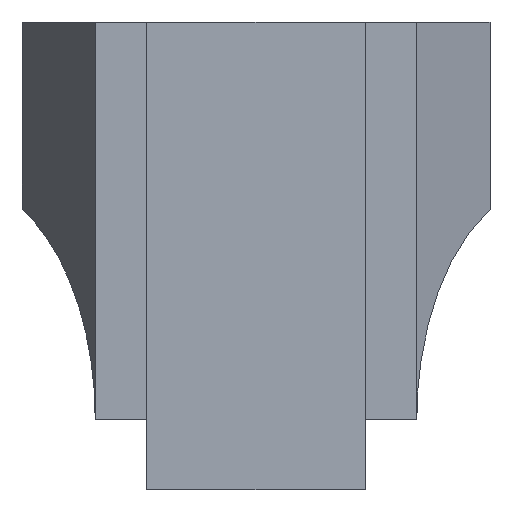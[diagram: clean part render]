
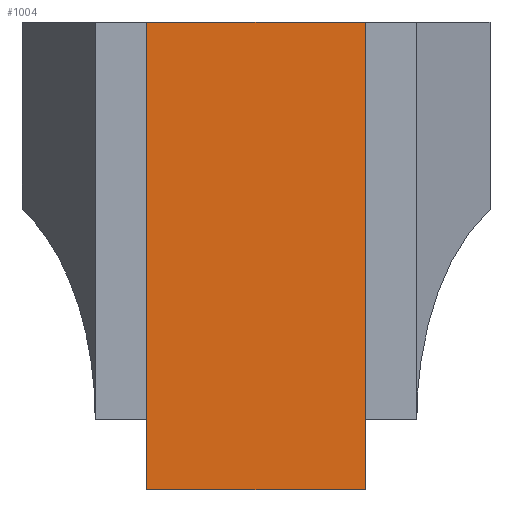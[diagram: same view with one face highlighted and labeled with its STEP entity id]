
A CAD part, front view. The second image highlights one B-rep face of the part: STEP entity #1004.
In plain terms, the highlighted planar face has unit normal (0, -1, 0).
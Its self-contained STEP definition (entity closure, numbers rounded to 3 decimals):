
#1004 = ADVANCED_FACE ( 'NONE', ( #13963 ), #10595, .T. ) ;
#1684 = CARTESIAN_POINT ( 'NONE',  ( 8.763, -36.779, -37.465 ) ) ;
#1995 = DIRECTION ( 'NONE',  ( 1., 0., 0. ) ) ;
#3786 = ORIENTED_EDGE ( 'NONE', *, *, #6204, .T. ) ;
#3848 = ORIENTED_EDGE ( 'NONE', *, *, #23478, .T. ) ;
#3893 = ORIENTED_EDGE ( 'NONE', *, *, #6611, .F. ) ;
#3922 = ORIENTED_EDGE ( 'NONE', *, *, #6567, .F. ) ;
#5533 = VECTOR ( 'NONE', #12416, 1000. ) ;
#5740 = EDGE_LOOP ( 'NONE', ( #3922, #3893, #3848, #3786 ) ) ;
#5918 = VERTEX_POINT ( 'NONE', #21819 ) ;
#6204 = EDGE_CURVE ( 'NONE', #5918, #16472, #19952, .T. ) ;
#6257 = VECTOR ( 'NONE', #18280, 1000. ) ;
#6567 = EDGE_CURVE ( 'NONE', #6609, #16472, #23216, .T. ) ;
#6609 = VERTEX_POINT ( 'NONE', #12443 ) ;
#6611 = EDGE_CURVE ( 'NONE', #12448, #6609, #9353, .T. ) ;
#9353 = LINE ( 'NONE', #12409, #25086 ) ;
#10561 = DIRECTION ( 'NONE',  ( 0., 0., -1. ) ) ;
#10587 = DIRECTION ( 'NONE',  ( 0., -1., 0. ) ) ;
#10595 = PLANE ( 'NONE',  #22796 ) ;
#10672 = CARTESIAN_POINT ( 'NONE',  ( 8.763, -36.779, -37.465 ) ) ;
#12132 = CARTESIAN_POINT ( 'NONE',  ( 8.763, -36.779, 0. ) ) ;
#12409 = CARTESIAN_POINT ( 'NONE',  ( -8.763, -36.779, -37.465 ) ) ;
#12416 = DIRECTION ( 'NONE',  ( 1., 0., 0. ) ) ;
#12443 = CARTESIAN_POINT ( 'NONE',  ( -8.763, -36.779, 0. ) ) ;
#12448 = VERTEX_POINT ( 'NONE', #17926 ) ;
#12679 = CARTESIAN_POINT ( 'NONE',  ( 8.763, -36.779, 0. ) ) ;
#13963 = FACE_OUTER_BOUND ( 'NONE', #5740, .T. ) ;
#14083 = LINE ( 'NONE', #26659, #16560 ) ;
#16472 = VERTEX_POINT ( 'NONE', #12132 ) ;
#16560 = VECTOR ( 'NONE', #1995, 1000. ) ;
#17926 = CARTESIAN_POINT ( 'NONE',  ( -8.763, -36.779, -37.465 ) ) ;
#18280 = DIRECTION ( 'NONE',  ( 0., 0., 1. ) ) ;
#19952 = LINE ( 'NONE', #1684, #6257 ) ;
#21819 = CARTESIAN_POINT ( 'NONE',  ( 8.763, -36.779, -37.465 ) ) ;
#22796 = AXIS2_PLACEMENT_3D ( 'NONE', #10672, #10587, #10561 ) ;
#23216 = LINE ( 'NONE', #12679, #5533 ) ;
#23478 = EDGE_CURVE ( 'NONE', #12448, #5918, #14083, .T. ) ;
#24293 = DIRECTION ( 'NONE',  ( 0., 0., 1. ) ) ;
#25086 = VECTOR ( 'NONE', #24293, 1000. ) ;
#26659 = CARTESIAN_POINT ( 'NONE',  ( 8.763, -36.779, -37.465 ) ) ;
